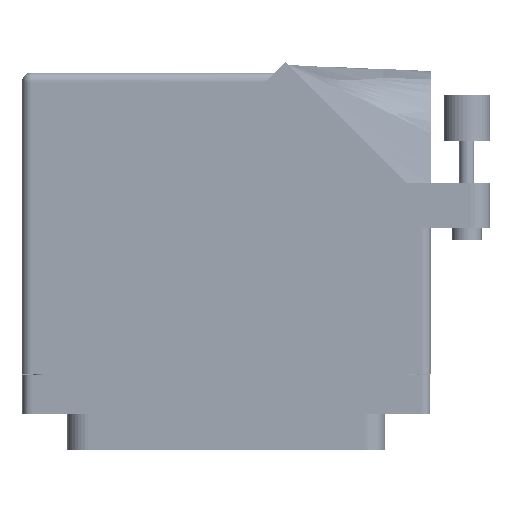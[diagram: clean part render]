
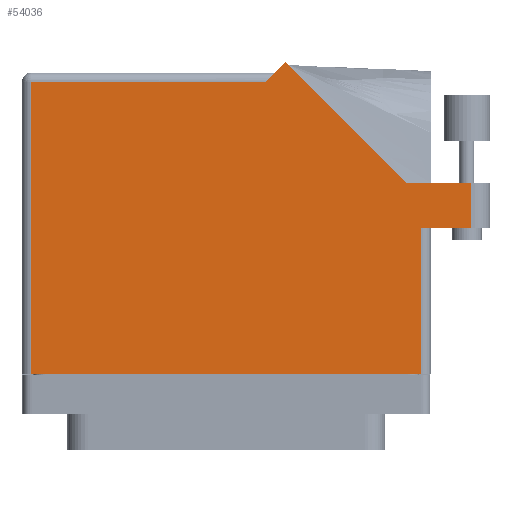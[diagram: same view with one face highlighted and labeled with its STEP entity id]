
A CAD part, front view. The second image highlights one B-rep face of the part: STEP entity #54036.
In plain terms, the highlighted face is planar.
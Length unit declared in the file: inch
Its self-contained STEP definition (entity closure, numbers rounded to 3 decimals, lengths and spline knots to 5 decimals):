
#933 = VECTOR ( 'NONE', #9768, 39.37008 ) ;
#3970 = LINE ( 'NONE', #30074, #30918 ) ;
#4186 = CARTESIAN_POINT ( 'NONE',  ( 1.3155, 0.88, 0.765 ) ) ;
#4506 = VECTOR ( 'NONE', #65547, 39.37008 ) ;
#5131 = CARTESIAN_POINT ( 'NONE',  ( -1.3155, 1.868, 0.765 ) ) ;
#8941 = LINE ( 'NONE', #73959, #33803 ) ;
#9768 = DIRECTION ( 'NONE',  ( -0.707, 0.707, 0. ) ) ;
#10170 = CARTESIAN_POINT ( 'NONE',  ( 1.3775, 0.88, 0.765 ) ) ;
#10830 = CARTESIAN_POINT ( 'NONE',  ( -1.3775, 1.93, 0.765 ) ) ;
#12563 = VECTOR ( 'NONE', #25223, 39.37008 ) ;
#12755 = EDGE_CURVE ( 'NONE', #56079, #61160, #36471, .T. ) ;
#13099 = LINE ( 'NONE', #10170, #4506 ) ;
#14214 = DIRECTION ( 'NONE',  ( 0., 1., 0. ) ) ;
#15048 = PLANE ( 'NONE',  #32970 ) ;
#18161 = VECTOR ( 'NONE', #14214, 39.37008 ) ;
#22480 = ORIENTED_EDGE ( 'NONE', *, *, #45743, .T. ) ;
#23055 = CARTESIAN_POINT ( 'NONE',  ( 1.21192, 1.187, 0.765 ) ) ;
#23775 = ORIENTED_EDGE ( 'NONE', *, *, #81133, .T. ) ;
#24243 = EDGE_CURVE ( 'NONE', #61160, #41292, #13099, .T. ) ;
#24300 = ORIENTED_EDGE ( 'NONE', *, *, #24243, .T. ) ;
#25223 = DIRECTION ( 'NONE',  ( 0., -1., 0. ) ) ;
#26095 = DIRECTION ( 'NONE',  ( -1., 0., 0. ) ) ;
#26290 = CARTESIAN_POINT ( 'NONE',  ( 0.3275, 1.93, 0.765 ) ) ;
#26662 = CARTESIAN_POINT ( 'NONE',  ( 1.7775, 1.187, 0.765 ) ) ;
#30074 = CARTESIAN_POINT ( 'NONE',  ( -1.3775, 1.868, 0.765 ) ) ;
#30464 = DIRECTION ( 'NONE',  ( 0., 0., -1. ) ) ;
#30918 = VECTOR ( 'NONE', #85213, 39.37008 ) ;
#30979 = DIRECTION ( 'NONE',  ( 0., 1., 0. ) ) ;
#32970 = AXIS2_PLACEMENT_3D ( 'NONE', #10830, #30464, #37617 ) ;
#33556 = VERTEX_POINT ( 'NONE', #45195 ) ;
#33803 = VECTOR ( 'NONE', #81489, 39.37008 ) ;
#34312 = CARTESIAN_POINT ( 'NONE',  ( 1.6525, 1.187, 0.765 ) ) ;
#35404 = EDGE_CURVE ( 'NONE', #71602, #33556, #74231, .T. ) ;
#35501 = CARTESIAN_POINT ( 'NONE',  ( -1.3155, -0.1, 0.765 ) ) ;
#36462 = EDGE_CURVE ( 'NONE', #73498, #84509, #3970, .T. ) ;
#36471 = LINE ( 'NONE', #48246, #18161 ) ;
#36581 = EDGE_CURVE ( 'NONE', #84509, #88304, #58825, .T. ) ;
#37617 = DIRECTION ( 'NONE',  ( -1., 0., 0. ) ) ;
#40799 = ORIENTED_EDGE ( 'NONE', *, *, #36462, .T. ) ;
#41292 = VERTEX_POINT ( 'NONE', #69119 ) ;
#45099 = LINE ( 'NONE', #34312, #75304 ) ;
#45195 = CARTESIAN_POINT ( 'NONE',  ( 0.39821, 2.00071, 0.765 ) ) ;
#45292 = EDGE_LOOP ( 'NONE', ( #24300, #23775, #62719, #72222, #22480, #40799, #89141, #60066, #58368 ) ) ;
#45743 = EDGE_CURVE ( 'NONE', #33556, #73498, #66378, .T. ) ;
#48246 = CARTESIAN_POINT ( 'NONE',  ( 1.3155, 0.88, 0.765 ) ) ;
#48355 = VERTEX_POINT ( 'NONE', #86540 ) ;
#50213 = CARTESIAN_POINT ( 'NONE',  ( 1.3155, -0.1, 0.765 ) ) ;
#52926 = LINE ( 'NONE', #26662, #64741 ) ;
#54036 = ADVANCED_FACE ( 'NONE', ( #71824 ), #15048, .F. ) ;
#54199 = DIRECTION ( 'NONE',  ( -0.707, -0.707, 0. ) ) ;
#56079 = VERTEX_POINT ( 'NONE', #50213 ) ;
#58368 = ORIENTED_EDGE ( 'NONE', *, *, #12755, .T. ) ;
#58825 = LINE ( 'NONE', #73436, #12563 ) ;
#60066 = ORIENTED_EDGE ( 'NONE', *, *, #73992, .T. ) ;
#61160 = VERTEX_POINT ( 'NONE', #4186 ) ;
#61856 = EDGE_CURVE ( 'NONE', #48355, #71602, #52926, .T. ) ;
#62719 = ORIENTED_EDGE ( 'NONE', *, *, #61856, .T. ) ;
#64741 = VECTOR ( 'NONE', #26095, 39.37008 ) ;
#65547 = DIRECTION ( 'NONE',  ( 1., 0., 0. ) ) ;
#66378 = LINE ( 'NONE', #26290, #68620 ) ;
#68620 = VECTOR ( 'NONE', #54199, 39.37008 ) ;
#69119 = CARTESIAN_POINT ( 'NONE',  ( 1.6525, 0.88, 0.765 ) ) ;
#71602 = VERTEX_POINT ( 'NONE', #86301 ) ;
#71824 = FACE_OUTER_BOUND ( 'NONE', #45292, .T. ) ;
#72222 = ORIENTED_EDGE ( 'NONE', *, *, #35404, .T. ) ;
#73436 = CARTESIAN_POINT ( 'NONE',  ( -1.3155, -0.1, 0.765 ) ) ;
#73498 = VERTEX_POINT ( 'NONE', #85273 ) ;
#73959 = CARTESIAN_POINT ( 'NONE',  ( -1.3775, -0.1, 0.765 ) ) ;
#73992 = EDGE_CURVE ( 'NONE', #88304, #56079, #8941, .T. ) ;
#74231 = LINE ( 'NONE', #23055, #933 ) ;
#75304 = VECTOR ( 'NONE', #30979, 39.37008 ) ;
#81133 = EDGE_CURVE ( 'NONE', #41292, #48355, #45099, .T. ) ;
#81489 = DIRECTION ( 'NONE',  ( 1., 0., 0. ) ) ;
#84509 = VERTEX_POINT ( 'NONE', #5131 ) ;
#85213 = DIRECTION ( 'NONE',  ( -1., 0., 0. ) ) ;
#85273 = CARTESIAN_POINT ( 'NONE',  ( 0.2655, 1.868, 0.765 ) ) ;
#86301 = CARTESIAN_POINT ( 'NONE',  ( 1.21192, 1.187, 0.765 ) ) ;
#86540 = CARTESIAN_POINT ( 'NONE',  ( 1.6525, 1.187, 0.765 ) ) ;
#88304 = VERTEX_POINT ( 'NONE', #35501 ) ;
#89141 = ORIENTED_EDGE ( 'NONE', *, *, #36581, .T. ) ;
